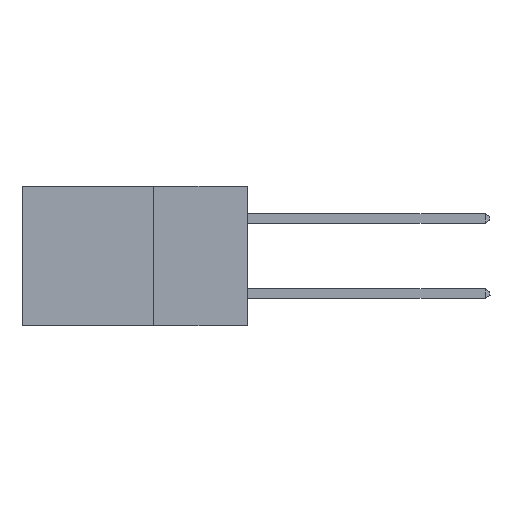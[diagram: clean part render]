
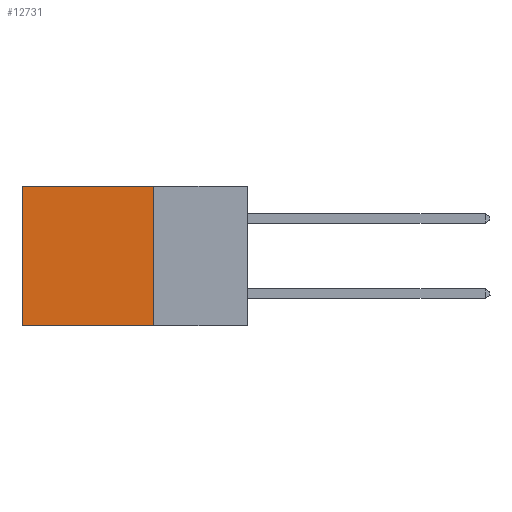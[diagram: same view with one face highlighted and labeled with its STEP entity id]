
A CAD part, left-side view. The second image highlights one B-rep face of the part: STEP entity #12731.
In plain terms, the highlighted planar face has unit normal (-1, 0, 0).
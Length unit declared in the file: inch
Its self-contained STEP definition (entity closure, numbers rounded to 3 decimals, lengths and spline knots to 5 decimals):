
#252 = VERTEX_POINT ( 'NONE', #11236 ) ;
#323 = CARTESIAN_POINT ( 'NONE',  ( 0.298, 0.6, 0. ) ) ;
#425 = CARTESIAN_POINT ( 'NONE',  ( 0.298, 0.6, 0. ) ) ;
#737 = CARTESIAN_POINT ( 'NONE',  ( 0.298, 0.25, 0. ) ) ;
#950 = CARTESIAN_POINT ( 'NONE',  ( 0.298, 0.25, -0.37 ) ) ;
#1413 = EDGE_CURVE ( 'NONE', #252, #9432, #12269, .T. ) ;
#1809 = VECTOR ( 'NONE', #7946, 39.37008 ) ;
#2114 = VECTOR ( 'NONE', #2708, 39.37008 ) ;
#2534 = FACE_OUTER_BOUND ( 'NONE', #6508, .T. ) ;
#2708 = DIRECTION ( 'NONE',  ( 0., 1., 0. ) ) ;
#2735 = DIRECTION ( 'NONE',  ( 0., 0., -1. ) ) ;
#3010 = VERTEX_POINT ( 'NONE', #11191 ) ;
#5338 = VECTOR ( 'NONE', #10153, 39.37008 ) ;
#5524 = CARTESIAN_POINT ( 'NONE',  ( 0.298, 0.25, 0. ) ) ;
#5686 = ORIENTED_EDGE ( 'NONE', *, *, #12547, .T. ) ;
#5727 = DIRECTION ( 'NONE',  ( 1., 0., 0. ) ) ;
#5841 = ORIENTED_EDGE ( 'NONE', *, *, #13714, .F. ) ;
#6508 = EDGE_LOOP ( 'NONE', ( #5686, #5841, #7977, #13150 ) ) ;
#7176 = VERTEX_POINT ( 'NONE', #950 ) ;
#7946 = DIRECTION ( 'NONE',  ( 0., 0., -1. ) ) ;
#7977 = ORIENTED_EDGE ( 'NONE', *, *, #12673, .F. ) ;
#9432 = VERTEX_POINT ( 'NONE', #425 ) ;
#10153 = DIRECTION ( 'NONE',  ( 0., 1., 0. ) ) ;
#10804 = LINE ( 'NONE', #323, #12103 ) ;
#10908 = LINE ( 'NONE', #13842, #1809 ) ;
#11191 = CARTESIAN_POINT ( 'NONE',  ( 0.298, 0.6, -0.37 ) ) ;
#11236 = CARTESIAN_POINT ( 'NONE',  ( 0.298, 0.25, 0. ) ) ;
#11403 = LINE ( 'NONE', #14338, #2114 ) ;
#11532 = PLANE ( 'NONE',  #13129 ) ;
#12103 = VECTOR ( 'NONE', #2735, 39.37008 ) ;
#12269 = LINE ( 'NONE', #737, #5338 ) ;
#12547 = EDGE_CURVE ( 'NONE', #9432, #3010, #10804, .T. ) ;
#12673 = EDGE_CURVE ( 'NONE', #252, #7176, #10908, .T. ) ;
#12731 = ADVANCED_FACE ( 'NONE', ( #2534 ), #11532, .F. ) ;
#13129 = AXIS2_PLACEMENT_3D ( 'NONE', #5524, #5727, #14834 ) ;
#13150 = ORIENTED_EDGE ( 'NONE', *, *, #1413, .T. ) ;
#13714 = EDGE_CURVE ( 'NONE', #7176, #3010, #11403, .T. ) ;
#13842 = CARTESIAN_POINT ( 'NONE',  ( 0.298, 0.25, 0. ) ) ;
#14338 = CARTESIAN_POINT ( 'NONE',  ( 0.298, 0.25, -0.37 ) ) ;
#14834 = DIRECTION ( 'NONE',  ( 0., 0., -1. ) ) ;
